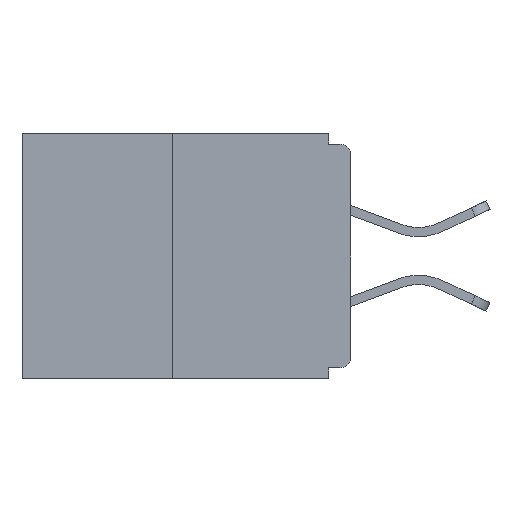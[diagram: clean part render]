
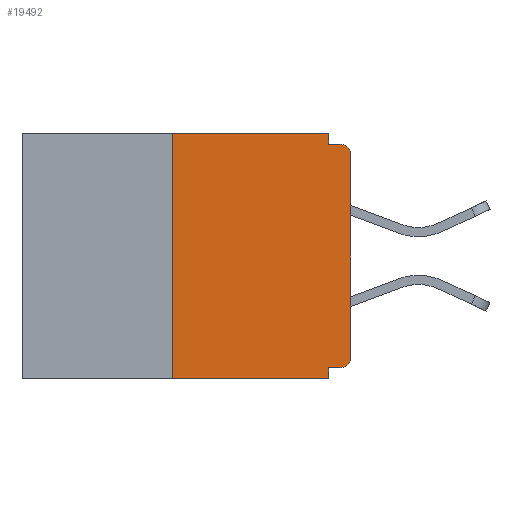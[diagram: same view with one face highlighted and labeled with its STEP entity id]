
A CAD part, left-side view. The second image highlights one B-rep face of the part: STEP entity #19492.
In plain terms, the highlighted planar face has unit normal (-1, 0, 0).
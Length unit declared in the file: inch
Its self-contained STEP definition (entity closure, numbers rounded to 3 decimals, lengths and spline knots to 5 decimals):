
#198 = EDGE_LOOP ( 'NONE', ( #17385, #3103, #24593, #5484, #23864, #4793, #26096, #22755, #20212, #13869 ) ) ;
#383 = EDGE_CURVE ( 'NONE', #20330, #973, #17347, .T. ) ;
#643 = EDGE_CURVE ( 'NONE', #12563, #15962, #6431, .T. ) ;
#675 = VERTEX_POINT ( 'NONE', #23483 ) ;
#791 = VERTEX_POINT ( 'NONE', #7716 ) ;
#973 = VERTEX_POINT ( 'NONE', #25150 ) ;
#1282 = CARTESIAN_POINT ( 'NONE',  ( 0., 0.25, 0. ) ) ;
#1393 = VECTOR ( 'NONE', #3762, 39.37008 ) ;
#2502 = CARTESIAN_POINT ( 'NONE',  ( 0., 0.25, 0. ) ) ;
#3103 = ORIENTED_EDGE ( 'NONE', *, *, #20064, .F. ) ;
#3120 = DIRECTION ( 'NONE',  ( -1., 0., 0. ) ) ;
#3187 = DIRECTION ( 'NONE',  ( 1., 0., 0. ) ) ;
#3207 = AXIS2_PLACEMENT_3D ( 'NONE', #22703, #24758, #4035 ) ;
#3634 = LINE ( 'NONE', #20157, #19094 ) ;
#3762 = DIRECTION ( 'NONE',  ( 0., 1., 0. ) ) ;
#3816 = VECTOR ( 'NONE', #12040, 39.37008 ) ;
#3940 = CARTESIAN_POINT ( 'NONE',  ( 0., 0., -0.328 ) ) ;
#3986 = CARTESIAN_POINT ( 'NONE',  ( 0., 0.031, -0.343 ) ) ;
#4035 = DIRECTION ( 'NONE',  ( 0., 0., -1. ) ) ;
#4194 = VECTOR ( 'NONE', #19998, 39.37008 ) ;
#4522 = VERTEX_POINT ( 'NONE', #12477 ) ;
#4793 = ORIENTED_EDGE ( 'NONE', *, *, #14537, .T. ) ;
#4944 = EDGE_CURVE ( 'NONE', #4522, #20330, #5819, .T. ) ;
#5039 = VECTOR ( 'NONE', #23902, 39.37008 ) ;
#5484 = ORIENTED_EDGE ( 'NONE', *, *, #17005, .F. ) ;
#5542 = DIRECTION ( 'NONE',  ( 0., 0., 1. ) ) ;
#5583 = DIRECTION ( 'NONE',  ( 0., 0., -1. ) ) ;
#5608 = EDGE_CURVE ( 'NONE', #19607, #973, #9650, .T. ) ;
#5774 = VECTOR ( 'NONE', #23306, 39.37008 ) ;
#5819 = LINE ( 'NONE', #20189, #4194 ) ;
#6431 = LINE ( 'NONE', #21222, #5774 ) ;
#6992 = AXIS2_PLACEMENT_3D ( 'NONE', #9618, #3187, #15538 ) ;
#7716 = CARTESIAN_POINT ( 'NONE',  ( 0., 0.031, 0. ) ) ;
#8231 = CIRCLE ( 'NONE', #10739, 0.015 ) ;
#9338 = CARTESIAN_POINT ( 'NONE',  ( 0., 0.031, -0.343 ) ) ;
#9618 = CARTESIAN_POINT ( 'NONE',  ( 0., 0.46, 0. ) ) ;
#9650 = LINE ( 'NONE', #9971, #3816 ) ;
#9971 = CARTESIAN_POINT ( 'NONE',  ( 0., 0., -0.015 ) ) ;
#10739 = AXIS2_PLACEMENT_3D ( 'NONE', #21877, #3120, #11632 ) ;
#11051 = VERTEX_POINT ( 'NONE', #2502 ) ;
#11632 = DIRECTION ( 'NONE',  ( 0., 0., -1. ) ) ;
#11894 = CARTESIAN_POINT ( 'NONE',  ( 0., 0.25, -0.343 ) ) ;
#12040 = DIRECTION ( 'NONE',  ( 0., -1., 0. ) ) ;
#12477 = CARTESIAN_POINT ( 'NONE',  ( 0., 0., -0.313 ) ) ;
#12563 = VERTEX_POINT ( 'NONE', #11894 ) ;
#12728 = VERTEX_POINT ( 'NONE', #21911 ) ;
#13869 = ORIENTED_EDGE ( 'NONE', *, *, #26337, .F. ) ;
#14537 = EDGE_CURVE ( 'NONE', #675, #4522, #8231, .T. ) ;
#15538 = DIRECTION ( 'NONE',  ( 0., 0., -1. ) ) ;
#15962 = VERTEX_POINT ( 'NONE', #3986 ) ;
#17005 = EDGE_CURVE ( 'NONE', #12728, #15962, #22115, .T. ) ;
#17347 = CIRCLE ( 'NONE', #3207, 0.015 ) ;
#17385 = ORIENTED_EDGE ( 'NONE', *, *, #22090, .F. ) ;
#17599 = LINE ( 'NONE', #18357, #22814 ) ;
#18357 = CARTESIAN_POINT ( 'NONE',  ( 0., 0.46, 0. ) ) ;
#18383 = EDGE_CURVE ( 'NONE', #675, #12728, #24939, .T. ) ;
#18753 = CARTESIAN_POINT ( 'NONE',  ( 0., 0., -0.03 ) ) ;
#19024 = LINE ( 'NONE', #1282, #24174 ) ;
#19094 = VECTOR ( 'NONE', #5583, 39.37008 ) ;
#19492 = ADVANCED_FACE ( 'NONE', ( #19669 ), #21757, .F. ) ;
#19607 = VERTEX_POINT ( 'NONE', #24277 ) ;
#19669 = FACE_OUTER_BOUND ( 'NONE', #198, .T. ) ;
#19998 = DIRECTION ( 'NONE',  ( 0., 0., 1. ) ) ;
#20064 = EDGE_CURVE ( 'NONE', #12563, #11051, #19024, .T. ) ;
#20157 = CARTESIAN_POINT ( 'NONE',  ( 0., 0.031, 0. ) ) ;
#20189 = CARTESIAN_POINT ( 'NONE',  ( 0., 0., 0. ) ) ;
#20212 = ORIENTED_EDGE ( 'NONE', *, *, #5608, .F. ) ;
#20330 = VERTEX_POINT ( 'NONE', #18753 ) ;
#21222 = CARTESIAN_POINT ( 'NONE',  ( 0., 0.46, -0.343 ) ) ;
#21757 = PLANE ( 'NONE',  #6992 ) ;
#21877 = CARTESIAN_POINT ( 'NONE',  ( 0., 0.015, -0.313 ) ) ;
#21911 = CARTESIAN_POINT ( 'NONE',  ( 0., 0.031, -0.328 ) ) ;
#22090 = EDGE_CURVE ( 'NONE', #11051, #791, #17599, .T. ) ;
#22115 = LINE ( 'NONE', #9338, #5039 ) ;
#22703 = CARTESIAN_POINT ( 'NONE',  ( 0., 0.015, -0.03 ) ) ;
#22755 = ORIENTED_EDGE ( 'NONE', *, *, #383, .T. ) ;
#22814 = VECTOR ( 'NONE', #26293, 39.37008 ) ;
#23306 = DIRECTION ( 'NONE',  ( 0., -1., 0. ) ) ;
#23483 = CARTESIAN_POINT ( 'NONE',  ( 0., 0.015, -0.328 ) ) ;
#23864 = ORIENTED_EDGE ( 'NONE', *, *, #18383, .F. ) ;
#23902 = DIRECTION ( 'NONE',  ( 0., 0., -1. ) ) ;
#24174 = VECTOR ( 'NONE', #5542, 39.37008 ) ;
#24277 = CARTESIAN_POINT ( 'NONE',  ( 0., 0.031, -0.015 ) ) ;
#24593 = ORIENTED_EDGE ( 'NONE', *, *, #643, .T. ) ;
#24758 = DIRECTION ( 'NONE',  ( -1., 0., 0. ) ) ;
#24939 = LINE ( 'NONE', #3940, #1393 ) ;
#25150 = CARTESIAN_POINT ( 'NONE',  ( 0., 0.015, -0.015 ) ) ;
#26096 = ORIENTED_EDGE ( 'NONE', *, *, #4944, .T. ) ;
#26293 = DIRECTION ( 'NONE',  ( 0., -1., 0. ) ) ;
#26337 = EDGE_CURVE ( 'NONE', #791, #19607, #3634, .T. ) ;
